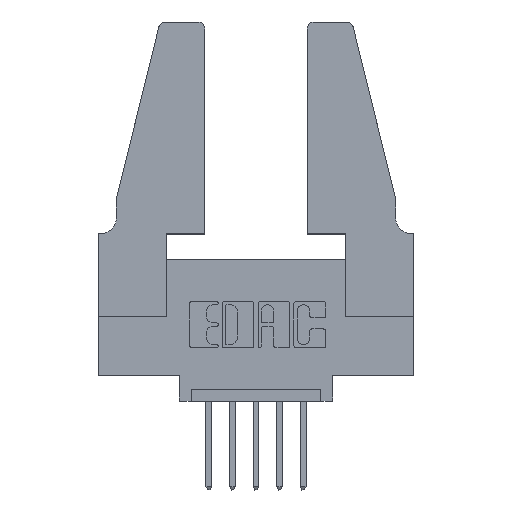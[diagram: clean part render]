
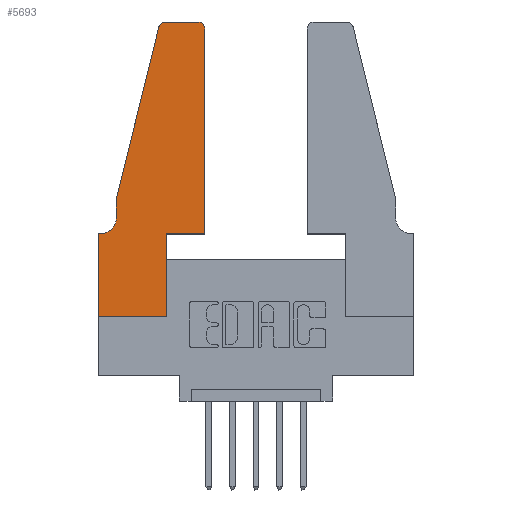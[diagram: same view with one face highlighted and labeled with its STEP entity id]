
A CAD part, top view. The second image highlights one B-rep face of the part: STEP entity #5693.
In plain terms, the highlighted planar face has unit normal (0, 0, 1).
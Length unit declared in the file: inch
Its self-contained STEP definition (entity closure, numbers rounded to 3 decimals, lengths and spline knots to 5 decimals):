
#227 = VERTEX_POINT ( 'NONE', #10518 ) ;
#384 = EDGE_CURVE ( 'NONE', #1398, #9546, #2573, .T. ) ;
#437 = DIRECTION ( 'NONE',  ( 0., 0., 1. ) ) ;
#493 = DIRECTION ( 'NONE',  ( -1., 0., 0. ) ) ;
#577 = VERTEX_POINT ( 'NONE', #9411 ) ;
#637 = CARTESIAN_POINT ( 'NONE',  ( 0.0055, 0.42, 0.37 ) ) ;
#663 = CARTESIAN_POINT ( 'NONE',  ( 0.0755, 0.5, 0.37 ) ) ;
#733 = VERTEX_POINT ( 'NONE', #1064 ) ;
#1064 = CARTESIAN_POINT ( 'NONE',  ( 0.0755, 0.42, 0.37 ) ) ;
#1082 = DIRECTION ( 'NONE',  ( 0., 0., 1. ) ) ;
#1278 = CARTESIAN_POINT ( 'NONE',  ( 0., 0., 0.37 ) ) ;
#1317 = CARTESIAN_POINT ( 'NONE',  ( 0.2865, 0., 0.37 ) ) ;
#1368 = CARTESIAN_POINT ( 'NONE',  ( 0.0755, 0.35, 0.37 ) ) ;
#1398 = VERTEX_POINT ( 'NONE', #8070 ) ;
#1424 = EDGE_CURVE ( 'NONE', #5169, #4463, #8280, .T. ) ;
#1544 = DIRECTION ( 'NONE',  ( -0.239, -0.971, 0. ) ) ;
#1600 = EDGE_CURVE ( 'NONE', #2885, #5169, #1993, .T. ) ;
#1650 = ORIENTED_EDGE ( 'NONE', *, *, #2762, .T. ) ;
#1695 = ORIENTED_EDGE ( 'NONE', *, *, #9210, .T. ) ;
#1825 = EDGE_CURVE ( 'NONE', #9546, #2885, #6922, .T. ) ;
#1890 = EDGE_LOOP ( 'NONE', ( #10840, #10195, #1650, #4527, #3282, #1695, #2793, #6731, #9633, #2334, #8936, #8183 ) ) ;
#1973 = CARTESIAN_POINT ( 'NONE',  ( 0.2865, 0.35, 0.37 ) ) ;
#1993 = LINE ( 'NONE', #10044, #6935 ) ;
#2242 = DIRECTION ( 'NONE',  ( 0., 0., -1. ) ) ;
#2303 = AXIS2_PLACEMENT_3D ( 'NONE', #6102, #1082, #2736 ) ;
#2334 = ORIENTED_EDGE ( 'NONE', *, *, #1600, .T. ) ;
#2368 = FACE_OUTER_BOUND ( 'NONE', #1890, .T. ) ;
#2573 = LINE ( 'NONE', #5799, #5249 ) ;
#2736 = DIRECTION ( 'NONE',  ( 1., 0., 0. ) ) ;
#2762 = EDGE_CURVE ( 'NONE', #577, #10974, #6097, .T. ) ;
#2793 = ORIENTED_EDGE ( 'NONE', *, *, #9766, .T. ) ;
#2797 = CARTESIAN_POINT ( 'NONE',  ( 0.0755, 0.5, 0.37 ) ) ;
#2885 = VERTEX_POINT ( 'NONE', #8302 ) ;
#3153 = VECTOR ( 'NONE', #3825, 39.37008 ) ;
#3154 = CARTESIAN_POINT ( 'NONE',  ( 0.0755, 0.5, 0.37 ) ) ;
#3282 = ORIENTED_EDGE ( 'NONE', *, *, #5878, .T. ) ;
#3676 = CARTESIAN_POINT ( 'NONE',  ( 0.4505, 0.35, 0.37 ) ) ;
#3812 = EDGE_CURVE ( 'NONE', #10974, #733, #4502, .T. ) ;
#3825 = DIRECTION ( 'NONE',  ( 0., -1., 0. ) ) ;
#3983 = DIRECTION ( 'NONE',  ( -1., 0., 0. ) ) ;
#4136 = DIRECTION ( 'NONE',  ( 1., 0., 0. ) ) ;
#4463 = VERTEX_POINT ( 'NONE', #10230 ) ;
#4502 = LINE ( 'NONE', #2797, #3153 ) ;
#4507 = EDGE_CURVE ( 'NONE', #7219, #577, #9748, .T. ) ;
#4525 = DIRECTION ( 'NONE',  ( 1., 0., 0. ) ) ;
#4527 = ORIENTED_EDGE ( 'NONE', *, *, #3812, .T. ) ;
#4532 = CIRCLE ( 'NONE', #6466, 0.03 ) ;
#4672 = DIRECTION ( 'NONE',  ( 0., -1., 0. ) ) ;
#4839 = VERTEX_POINT ( 'NONE', #10155 ) ;
#4851 = CARTESIAN_POINT ( 'NONE',  ( 0.4505, 0.35, 0.37 ) ) ;
#5169 = VERTEX_POINT ( 'NONE', #3676 ) ;
#5249 = VECTOR ( 'NONE', #4136, 39.37008 ) ;
#5396 = VECTOR ( 'NONE', #7359, 39.37008 ) ;
#5549 = CARTESIAN_POINT ( 'NONE',  ( 0.4205, 1.22, 0.37 ) ) ;
#5693 = ADVANCED_FACE ( 'NONE', ( #2368 ), #10340, .T. ) ;
#5782 = LINE ( 'NONE', #10836, #5396 ) ;
#5799 = CARTESIAN_POINT ( 'NONE',  ( 0., 0., 0.37 ) ) ;
#5878 = EDGE_CURVE ( 'NONE', #733, #9497, #7162, .T. ) ;
#5952 = AXIS2_PLACEMENT_3D ( 'NONE', #637, #2242, #493 ) ;
#5989 = VECTOR ( 'NONE', #7161, 39.37008 ) ;
#6097 = LINE ( 'NONE', #3154, #10517 ) ;
#6102 = CARTESIAN_POINT ( 'NONE',  ( 0.284, 1.22, 0.37 ) ) ;
#6142 = CARTESIAN_POINT ( 'NONE',  ( 0., 0.35, 0.37 ) ) ;
#6225 = CARTESIAN_POINT ( 'NONE',  ( 0.284, 1.25, 0.37 ) ) ;
#6466 = AXIS2_PLACEMENT_3D ( 'NONE', #5549, #437, #8272 ) ;
#6731 = ORIENTED_EDGE ( 'NONE', *, *, #384, .T. ) ;
#6922 = LINE ( 'NONE', #1973, #8136 ) ;
#6935 = VECTOR ( 'NONE', #11066, 39.37008 ) ;
#6944 = LINE ( 'NONE', #1368, #10822 ) ;
#7044 = DIRECTION ( 'NONE',  ( 0., 0., 1. ) ) ;
#7161 = DIRECTION ( 'NONE',  ( 0., 1., 0. ) ) ;
#7162 = CIRCLE ( 'NONE', #5952, 0.07 ) ;
#7219 = VERTEX_POINT ( 'NONE', #6225 ) ;
#7359 = DIRECTION ( 'NONE',  ( -1., 0., 0. ) ) ;
#7479 = EDGE_CURVE ( 'NONE', #4839, #7219, #5782, .T. ) ;
#7994 = DIRECTION ( 'NONE',  ( 0., 1., 0. ) ) ;
#8070 = CARTESIAN_POINT ( 'NONE',  ( 0., 0., 0.37 ) ) ;
#8136 = VECTOR ( 'NONE', #7994, 39.37008 ) ;
#8183 = ORIENTED_EDGE ( 'NONE', *, *, #10394, .T. ) ;
#8272 = DIRECTION ( 'NONE',  ( 1., 0., 0. ) ) ;
#8280 = LINE ( 'NONE', #4851, #5989 ) ;
#8302 = CARTESIAN_POINT ( 'NONE',  ( 0.2865, 0.35, 0.37 ) ) ;
#8936 = ORIENTED_EDGE ( 'NONE', *, *, #1424, .T. ) ;
#8959 = LINE ( 'NONE', #1278, #9896 ) ;
#9025 = CARTESIAN_POINT ( 'NONE',  ( 0.0055, 0.35, 0.37 ) ) ;
#9210 = EDGE_CURVE ( 'NONE', #9497, #227, #6944, .T. ) ;
#9261 = AXIS2_PLACEMENT_3D ( 'NONE', #6142, #7044, #4525 ) ;
#9411 = CARTESIAN_POINT ( 'NONE',  ( 0.25487, 1.22718, 0.37 ) ) ;
#9497 = VERTEX_POINT ( 'NONE', #9025 ) ;
#9546 = VERTEX_POINT ( 'NONE', #1317 ) ;
#9633 = ORIENTED_EDGE ( 'NONE', *, *, #1825, .T. ) ;
#9748 = CIRCLE ( 'NONE', #2303, 0.03 ) ;
#9766 = EDGE_CURVE ( 'NONE', #227, #1398, #8959, .T. ) ;
#9896 = VECTOR ( 'NONE', #4672, 39.37008 ) ;
#10044 = CARTESIAN_POINT ( 'NONE',  ( 0.4505, 0.35, 0.37 ) ) ;
#10155 = CARTESIAN_POINT ( 'NONE',  ( 0.4205, 1.25, 0.37 ) ) ;
#10195 = ORIENTED_EDGE ( 'NONE', *, *, #4507, .T. ) ;
#10230 = CARTESIAN_POINT ( 'NONE',  ( 0.4505, 1.22, 0.37 ) ) ;
#10340 = PLANE ( 'NONE',  #9261 ) ;
#10394 = EDGE_CURVE ( 'NONE', #4463, #4839, #4532, .T. ) ;
#10517 = VECTOR ( 'NONE', #1544, 39.37008 ) ;
#10518 = CARTESIAN_POINT ( 'NONE',  ( 0., 0.35, 0.37 ) ) ;
#10822 = VECTOR ( 'NONE', #3983, 39.37008 ) ;
#10836 = CARTESIAN_POINT ( 'NONE',  ( 0.2605, 1.25, 0.37 ) ) ;
#10840 = ORIENTED_EDGE ( 'NONE', *, *, #7479, .T. ) ;
#10974 = VERTEX_POINT ( 'NONE', #663 ) ;
#11066 = DIRECTION ( 'NONE',  ( 1., 0., 0. ) ) ;
